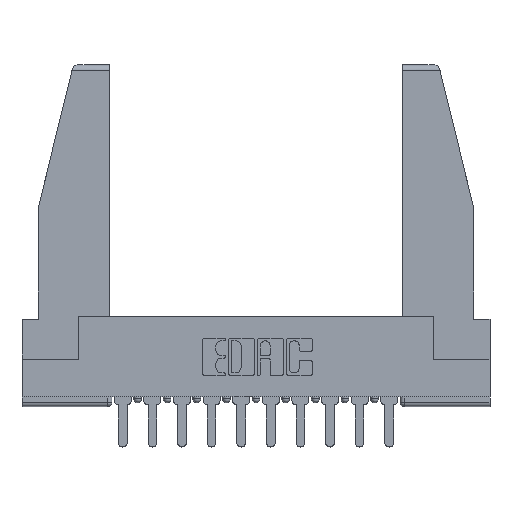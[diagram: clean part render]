
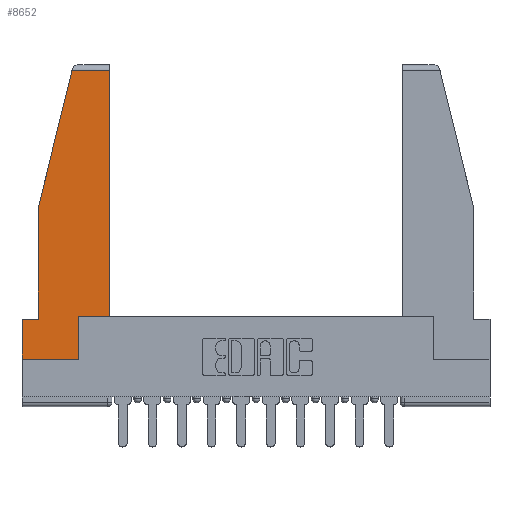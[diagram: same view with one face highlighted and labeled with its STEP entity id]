
A CAD part, top view. The second image highlights one B-rep face of the part: STEP entity #8652.
In plain terms, the highlighted planar face has unit normal (0, 0, 1).
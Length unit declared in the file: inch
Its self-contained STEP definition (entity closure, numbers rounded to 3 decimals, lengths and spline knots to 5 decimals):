
#31 = ORIENTED_EDGE ( 'NONE', *, *, #1855, .T. ) ;
#674 = VERTEX_POINT ( 'NONE', #10421 ) ;
#784 = ORIENTED_EDGE ( 'NONE', *, *, #10568, .T. ) ;
#896 = LINE ( 'NONE', #7580, #11900 ) ;
#901 = CARTESIAN_POINT ( 'NONE',  ( 0.086, 0.8, 0. ) ) ;
#1310 = LINE ( 'NONE', #9594, #5130 ) ;
#1379 = DIRECTION ( 'NONE',  ( 0., 1., 0. ) ) ;
#1412 = CARTESIAN_POINT ( 'NONE',  ( 0.297, 0.223, 0. ) ) ;
#1694 = ORIENTED_EDGE ( 'NONE', *, *, #4058, .T. ) ;
#1855 = EDGE_CURVE ( 'NONE', #12593, #7535, #10981, .T. ) ;
#2026 = ORIENTED_EDGE ( 'NONE', *, *, #5071, .T. ) ;
#2711 = LINE ( 'NONE', #7284, #7655 ) ;
#2966 = CARTESIAN_POINT ( 'NONE',  ( 0., 0.21, 0. ) ) ;
#3042 = ORIENTED_EDGE ( 'NONE', *, *, #3334, .T. ) ;
#3334 = EDGE_CURVE ( 'NONE', #12402, #15147, #5667, .T. ) ;
#3469 = DIRECTION ( 'NONE',  ( 0., 0., 1. ) ) ;
#3523 = VECTOR ( 'NONE', #5768, 39.37008 ) ;
#3560 = AXIS2_PLACEMENT_3D ( 'NONE', #12791, #3469, #14135 ) ;
#3632 = DIRECTION ( 'NONE',  ( 1., 0., 0. ) ) ;
#3679 = VECTOR ( 'NONE', #9868, 39.37008 ) ;
#3792 = CARTESIAN_POINT ( 'NONE',  ( 0.461, 0.223, 0. ) ) ;
#3926 = CARTESIAN_POINT ( 'NONE',  ( 0.086, 0.8, 0. ) ) ;
#4058 = EDGE_CURVE ( 'NONE', #15147, #13864, #13350, .T. ) ;
#4560 = EDGE_CURVE ( 'NONE', #7535, #12402, #2711, .T. ) ;
#4903 = ORIENTED_EDGE ( 'NONE', *, *, #12382, .T. ) ;
#5071 = EDGE_CURVE ( 'NONE', #13864, #11591, #896, .T. ) ;
#5130 = VECTOR ( 'NONE', #1379, 39.37008 ) ;
#5510 = DIRECTION ( 'NONE',  ( 0., -1., 0. ) ) ;
#5586 = DIRECTION ( 'NONE',  ( 0., -1., 0. ) ) ;
#5667 = LINE ( 'NONE', #901, #12737 ) ;
#5768 = DIRECTION ( 'NONE',  ( 1., 0., 0. ) ) ;
#6010 = EDGE_CURVE ( 'NONE', #11591, #11838, #15050, .T. ) ;
#6074 = LINE ( 'NONE', #14361, #10038 ) ;
#6474 = VECTOR ( 'NONE', #7339, 39.37008 ) ;
#6845 = PLANE ( 'NONE',  #3560 ) ;
#7284 = CARTESIAN_POINT ( 'NONE',  ( 0.271, 1.55, 0. ) ) ;
#7339 = DIRECTION ( 'NONE',  ( -1., 0., 0. ) ) ;
#7535 = VERTEX_POINT ( 'NONE', #10779 ) ;
#7580 = CARTESIAN_POINT ( 'NONE',  ( 0., 0.21, 0. ) ) ;
#7655 = VECTOR ( 'NONE', #8686, 39.37008 ) ;
#8392 = LINE ( 'NONE', #1412, #14254 ) ;
#8652 = ADVANCED_FACE ( 'NONE', ( #10562 ), #6845, .T. ) ;
#8686 = DIRECTION ( 'NONE',  ( -0.239, -0.971, 0. ) ) ;
#9366 = ORIENTED_EDGE ( 'NONE', *, *, #6010, .T. ) ;
#9594 = CARTESIAN_POINT ( 'NONE',  ( 0.297, 0., 0. ) ) ;
#9651 = CARTESIAN_POINT ( 'NONE',  ( 0.297, 0., 0. ) ) ;
#9868 = DIRECTION ( 'NONE',  ( -1., 0., 0. ) ) ;
#9912 = CARTESIAN_POINT ( 'NONE',  ( 0., 0., 0. ) ) ;
#10038 = VECTOR ( 'NONE', #11004, 39.37008 ) ;
#10421 = CARTESIAN_POINT ( 'NONE',  ( 0.297, 0.223, 0. ) ) ;
#10562 = FACE_OUTER_BOUND ( 'NONE', #13223, .T. ) ;
#10568 = EDGE_CURVE ( 'NONE', #674, #10574, #8392, .T. ) ;
#10574 = VERTEX_POINT ( 'NONE', #3792 ) ;
#10779 = CARTESIAN_POINT ( 'NONE',  ( 0.2636, 1.52, 0. ) ) ;
#10981 = LINE ( 'NONE', #11065, #6474 ) ;
#11004 = DIRECTION ( 'NONE',  ( 0., 1., 0. ) ) ;
#11065 = CARTESIAN_POINT ( 'NONE',  ( 0., 1.52, 0. ) ) ;
#11591 = VERTEX_POINT ( 'NONE', #9912 ) ;
#11838 = VERTEX_POINT ( 'NONE', #9651 ) ;
#11900 = VECTOR ( 'NONE', #5510, 39.37008 ) ;
#11965 = CARTESIAN_POINT ( 'NONE',  ( 0., 0.21, 0. ) ) ;
#12322 = ORIENTED_EDGE ( 'NONE', *, *, #12639, .T. ) ;
#12382 = EDGE_CURVE ( 'NONE', #10574, #12593, #6074, .T. ) ;
#12402 = VERTEX_POINT ( 'NONE', #3926 ) ;
#12593 = VERTEX_POINT ( 'NONE', #12852 ) ;
#12639 = EDGE_CURVE ( 'NONE', #11838, #674, #1310, .T. ) ;
#12737 = VECTOR ( 'NONE', #5586, 39.37008 ) ;
#12791 = CARTESIAN_POINT ( 'NONE',  ( 0., 0., 0. ) ) ;
#12852 = CARTESIAN_POINT ( 'NONE',  ( 0.461, 1.52, 0. ) ) ;
#13223 = EDGE_LOOP ( 'NONE', ( #4903, #31, #13867, #3042, #1694, #2026, #9366, #12322, #784 ) ) ;
#13350 = LINE ( 'NONE', #11965, #3679 ) ;
#13810 = CARTESIAN_POINT ( 'NONE',  ( 0., 0., 0. ) ) ;
#13864 = VERTEX_POINT ( 'NONE', #2966 ) ;
#13867 = ORIENTED_EDGE ( 'NONE', *, *, #4560, .T. ) ;
#14135 = DIRECTION ( 'NONE',  ( 1., 0., 0. ) ) ;
#14254 = VECTOR ( 'NONE', #3632, 39.37008 ) ;
#14361 = CARTESIAN_POINT ( 'NONE',  ( 0.461, 0.223, 0. ) ) ;
#14763 = CARTESIAN_POINT ( 'NONE',  ( 0.086, 0.21, 0. ) ) ;
#15050 = LINE ( 'NONE', #13810, #3523 ) ;
#15147 = VERTEX_POINT ( 'NONE', #14763 ) ;
